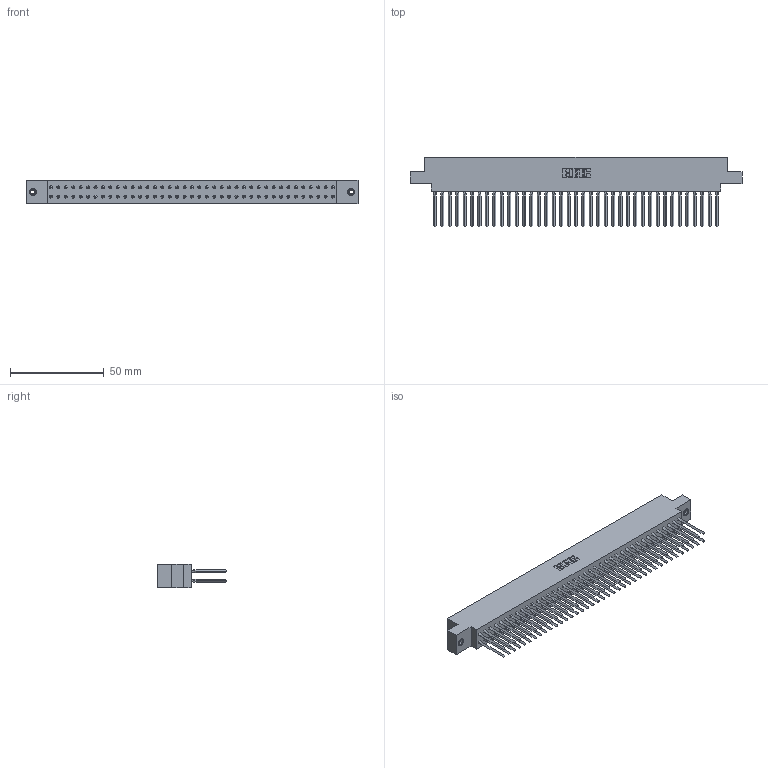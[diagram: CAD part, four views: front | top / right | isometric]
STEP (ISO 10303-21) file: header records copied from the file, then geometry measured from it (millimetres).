
FILE_DESCRIPTION (( 'STEP AP203' ), '1' );
FILE_NAME ('317-078-540-808.STEP', '2020-02-28T08:44:08', ( '' ), ( '' ), 'SwSTEP 2.0', 'SolidWorks 2016', '' );
FILE_SCHEMA (( 'CONFIG_CONTROL_DESIGN' ));
Length unit declared in the file: inch
Products named in the file (4): 345-250-001_345-250-003-102; 317 Part_.156 Dia - TI; 317-290-001_540; 317-078-540-808
Assembly tree (81 placements, depth 2):
  317-078-540-808
    317 Part_.156 Dia - TI
    317-290-001_540  x78
    345-250-001_345-250-003-102  x2
Bounding box: 177.24 x 37.34 x 12.7 mm (x, y, z)
Volume: 29638.6 mm3; surface area: 44097.6 mm2
Topology: 81 solids, 81 shells, 7104 faces, 19677 edges, 12668 vertices
Faces by surface type: plane 5784, cylinder 992, bspline 312, cone 12, torus 4
Entity records: 57979 total; most frequent: CARTESIAN_POINT 10502, ORIENTED_EDGE 9994, DIRECTION 8377, EDGE_CURVE 4997, LINE 4721, VECTOR 4721, VERTEX_POINT 3321, AXIS2_PLACEMENT_3D 1828
